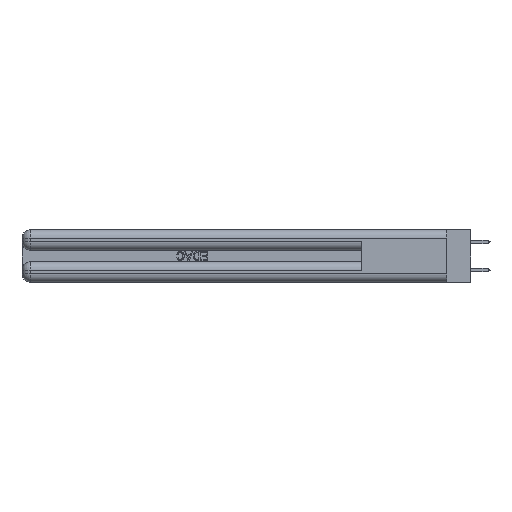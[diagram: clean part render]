
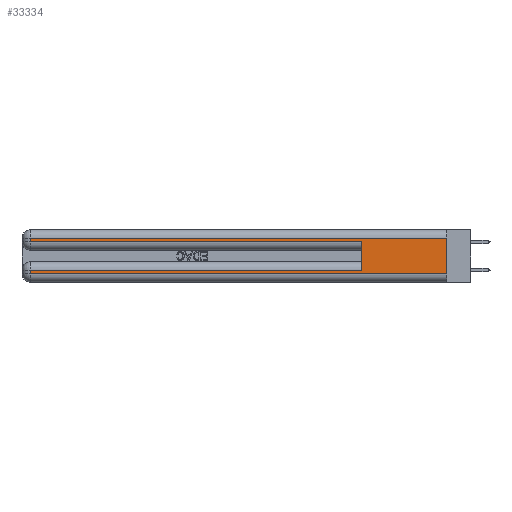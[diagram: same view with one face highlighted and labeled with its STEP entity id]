
A CAD part, left-side view. The second image highlights one B-rep face of the part: STEP entity #33334.
In plain terms, the highlighted planar face has unit normal (-1, 0, 0).
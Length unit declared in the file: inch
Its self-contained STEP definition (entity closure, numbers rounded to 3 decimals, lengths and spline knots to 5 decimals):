
#2372 = VECTOR ( 'NONE', #34554, 39.37008 ) ;
#2412 = DIRECTION ( 'NONE',  ( 0., 0., -1. ) ) ;
#3553 = VERTEX_POINT ( 'NONE', #39458 ) ;
#3568 = EDGE_CURVE ( 'NONE', #3553, #33600, #46738, .T. ) ;
#3773 = VECTOR ( 'NONE', #36811, 39.37008 ) ;
#4158 = PLANE ( 'NONE',  #26048 ) ;
#4419 = CARTESIAN_POINT ( 'NONE',  ( 0., 0., 0.285 ) ) ;
#4489 = DIRECTION ( 'NONE',  ( 0., 0., -1. ) ) ;
#4570 = DIRECTION ( 'NONE',  ( 0., 1., 0. ) ) ;
#5073 = CARTESIAN_POINT ( 'NONE',  ( 0., 2.94, 0.37 ) ) ;
#6367 = ORIENTED_EDGE ( 'NONE', *, *, #25815, .T. ) ;
#6575 = CARTESIAN_POINT ( 'NONE',  ( 0., 2.94, 0.37 ) ) ;
#6784 = CARTESIAN_POINT ( 'NONE',  ( 0., 0.6, 0.145 ) ) ;
#7542 = CARTESIAN_POINT ( 'NONE',  ( 0., 0., 0.06 ) ) ;
#7801 = ORIENTED_EDGE ( 'NONE', *, *, #8902, .F. ) ;
#7934 = LINE ( 'NONE', #10002, #25106 ) ;
#8838 = ORIENTED_EDGE ( 'NONE', *, *, #15258, .T. ) ;
#8902 = EDGE_CURVE ( 'NONE', #17304, #10784, #10733, .T. ) ;
#10002 = CARTESIAN_POINT ( 'NONE',  ( 0., 0., 0.085 ) ) ;
#10733 = LINE ( 'NONE', #38308, #31367 ) ;
#10784 = VERTEX_POINT ( 'NONE', #43877 ) ;
#11341 = DIRECTION ( 'NONE',  ( 0., -1., 0. ) ) ;
#11839 = ORIENTED_EDGE ( 'NONE', *, *, #47161, .T. ) ;
#13214 = EDGE_CURVE ( 'NONE', #33600, #31342, #17201, .T. ) ;
#14372 = EDGE_LOOP ( 'NONE', ( #7801, #11839, #42478, #41324, #35950, #26233, #8838, #6367 ) ) ;
#15258 = EDGE_CURVE ( 'NONE', #29050, #46009, #36883, .T. ) ;
#15628 = FACE_OUTER_BOUND ( 'NONE', #14372, .T. ) ;
#15920 = CARTESIAN_POINT ( 'NONE',  ( 0., 0., 0.37 ) ) ;
#16442 = VECTOR ( 'NONE', #11341, 39.37008 ) ;
#17201 = LINE ( 'NONE', #4419, #2372 ) ;
#17304 = VERTEX_POINT ( 'NONE', #19192 ) ;
#17516 = VECTOR ( 'NONE', #38325, 39.37008 ) ;
#17569 = CARTESIAN_POINT ( 'NONE',  ( 0., 2.94, 0.285 ) ) ;
#18434 = CARTESIAN_POINT ( 'NONE',  ( 0., 0.6, 0.285 ) ) ;
#19192 = CARTESIAN_POINT ( 'NONE',  ( 0., 0., 0.31 ) ) ;
#19393 = CARTESIAN_POINT ( 'NONE',  ( 0., 2.94, 0.06 ) ) ;
#23701 = EDGE_CURVE ( 'NONE', #33979, #29050, #7934, .T. ) ;
#23917 = CARTESIAN_POINT ( 'NONE',  ( 0., 2.94, 0.085 ) ) ;
#25076 = DIRECTION ( 'NONE',  ( 0., 1., 0. ) ) ;
#25106 = VECTOR ( 'NONE', #25076, 39.37008 ) ;
#25622 = DIRECTION ( 'NONE',  ( 0., 0., 1. ) ) ;
#25815 = EDGE_CURVE ( 'NONE', #46009, #10784, #26457, .T. ) ;
#26048 = AXIS2_PLACEMENT_3D ( 'NONE', #15920, #34789, #4489 ) ;
#26233 = ORIENTED_EDGE ( 'NONE', *, *, #23701, .T. ) ;
#26457 = LINE ( 'NONE', #7542, #16442 ) ;
#29050 = VERTEX_POINT ( 'NONE', #23917 ) ;
#29958 = CARTESIAN_POINT ( 'NONE',  ( 0., 0., 0.31 ) ) ;
#31066 = VECTOR ( 'NONE', #25622, 39.37008 ) ;
#31342 = VERTEX_POINT ( 'NONE', #18434 ) ;
#31367 = VECTOR ( 'NONE', #2412, 39.37008 ) ;
#33334 = ADVANCED_FACE ( 'NONE', ( #15628 ), #4158, .F. ) ;
#33600 = VERTEX_POINT ( 'NONE', #17569 ) ;
#33979 = VERTEX_POINT ( 'NONE', #45643 ) ;
#34554 = DIRECTION ( 'NONE',  ( 0., -1., 0. ) ) ;
#34789 = DIRECTION ( 'NONE',  ( 1., 0., 0. ) ) ;
#35186 = LINE ( 'NONE', #29958, #36353 ) ;
#35950 = ORIENTED_EDGE ( 'NONE', *, *, #43675, .F. ) ;
#36353 = VECTOR ( 'NONE', #4570, 39.37008 ) ;
#36811 = DIRECTION ( 'NONE',  ( 0., 0., -1. ) ) ;
#36883 = LINE ( 'NONE', #5073, #17516 ) ;
#38308 = CARTESIAN_POINT ( 'NONE',  ( 0., 0., 0.37 ) ) ;
#38325 = DIRECTION ( 'NONE',  ( 0., 0., -1. ) ) ;
#39458 = CARTESIAN_POINT ( 'NONE',  ( 0., 2.94, 0.31 ) ) ;
#41324 = ORIENTED_EDGE ( 'NONE', *, *, #13214, .T. ) ;
#42478 = ORIENTED_EDGE ( 'NONE', *, *, #3568, .T. ) ;
#43675 = EDGE_CURVE ( 'NONE', #33979, #31342, #47471, .T. ) ;
#43877 = CARTESIAN_POINT ( 'NONE',  ( 0., 0., 0.06 ) ) ;
#45643 = CARTESIAN_POINT ( 'NONE',  ( 0., 0.6, 0.085 ) ) ;
#46009 = VERTEX_POINT ( 'NONE', #19393 ) ;
#46738 = LINE ( 'NONE', #6575, #3773 ) ;
#47161 = EDGE_CURVE ( 'NONE', #17304, #3553, #35186, .T. ) ;
#47471 = LINE ( 'NONE', #6784, #31066 ) ;
